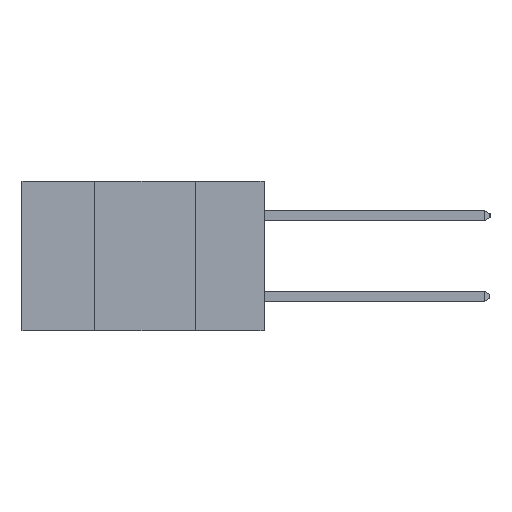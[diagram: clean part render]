
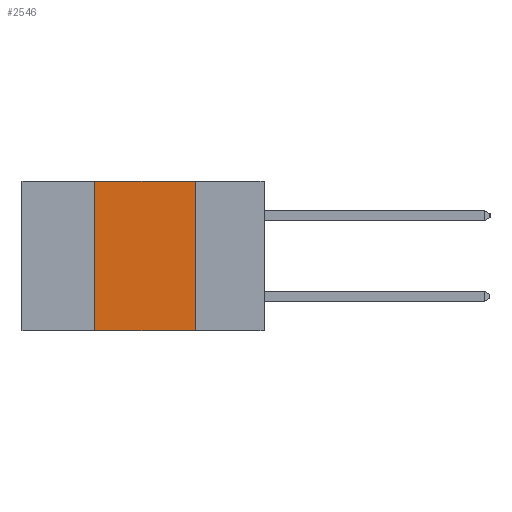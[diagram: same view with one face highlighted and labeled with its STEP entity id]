
A CAD part, left-side view. The second image highlights one B-rep face of the part: STEP entity #2546.
In plain terms, the highlighted planar face has unit normal (-1, 0, 0).
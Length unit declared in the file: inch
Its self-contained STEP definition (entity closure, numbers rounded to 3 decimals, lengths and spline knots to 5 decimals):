
#1181 = LINE ( 'NONE', #2153, #12783 ) ;
#1298 = ORIENTED_EDGE ( 'NONE', *, *, #3796, .F. ) ;
#2006 = DIRECTION ( 'NONE',  ( 0., 0., 1. ) ) ;
#2153 = CARTESIAN_POINT ( 'NONE',  ( 0., 0.6, -0.37 ) ) ;
#2188 = EDGE_CURVE ( 'NONE', #3852, #6266, #12042, .T. ) ;
#2546 = ADVANCED_FACE ( 'NONE', ( #2971 ), #9832, .F. ) ;
#2585 = ORIENTED_EDGE ( 'NONE', *, *, #8984, .T. ) ;
#2803 = CARTESIAN_POINT ( 'NONE',  ( 0., 0.42, 0. ) ) ;
#2971 = FACE_OUTER_BOUND ( 'NONE', #11895, .T. ) ;
#2972 = DIRECTION ( 'NONE',  ( 0., -1., 0. ) ) ;
#3703 = CARTESIAN_POINT ( 'NONE',  ( 0., 0.42, -0.37 ) ) ;
#3796 = EDGE_CURVE ( 'NONE', #11237, #3852, #7047, .T. ) ;
#3852 = VERTEX_POINT ( 'NONE', #3928 ) ;
#3928 = CARTESIAN_POINT ( 'NONE',  ( 0., 0.17, 0. ) ) ;
#3944 = CARTESIAN_POINT ( 'NONE',  ( 0., 0.17, -0.37 ) ) ;
#3990 = DIRECTION ( 'NONE',  ( 0., 0., -1. ) ) ;
#5098 = CARTESIAN_POINT ( 'NONE',  ( 0., 0.6, 0. ) ) ;
#5107 = VECTOR ( 'NONE', #2972, 39.37008 ) ;
#6006 = DIRECTION ( 'NONE',  ( 0., -1., 0. ) ) ;
#6266 = VERTEX_POINT ( 'NONE', #7086 ) ;
#6678 = AXIS2_PLACEMENT_3D ( 'NONE', #6788, #10017, #3990 ) ;
#6788 = CARTESIAN_POINT ( 'NONE',  ( 0., 0.6, 0. ) ) ;
#6951 = LINE ( 'NONE', #3703, #12789 ) ;
#7047 = LINE ( 'NONE', #5098, #5107 ) ;
#7086 = CARTESIAN_POINT ( 'NONE',  ( 0., 0.17, -0.37 ) ) ;
#7243 = DIRECTION ( 'NONE',  ( 0., 0., -1. ) ) ;
#8660 = ORIENTED_EDGE ( 'NONE', *, *, #11277, .F. ) ;
#8984 = EDGE_CURVE ( 'NONE', #10802, #6266, #1181, .T. ) ;
#9121 = VECTOR ( 'NONE', #7243, 39.37008 ) ;
#9825 = ORIENTED_EDGE ( 'NONE', *, *, #2188, .F. ) ;
#9832 = PLANE ( 'NONE',  #6678 ) ;
#10017 = DIRECTION ( 'NONE',  ( 1., 0., 0. ) ) ;
#10802 = VERTEX_POINT ( 'NONE', #12675 ) ;
#11237 = VERTEX_POINT ( 'NONE', #2803 ) ;
#11277 = EDGE_CURVE ( 'NONE', #10802, #11237, #6951, .T. ) ;
#11895 = EDGE_LOOP ( 'NONE', ( #9825, #1298, #8660, #2585 ) ) ;
#12042 = LINE ( 'NONE', #3944, #9121 ) ;
#12675 = CARTESIAN_POINT ( 'NONE',  ( 0., 0.42, -0.37 ) ) ;
#12783 = VECTOR ( 'NONE', #6006, 39.37008 ) ;
#12789 = VECTOR ( 'NONE', #2006, 39.37008 ) ;
